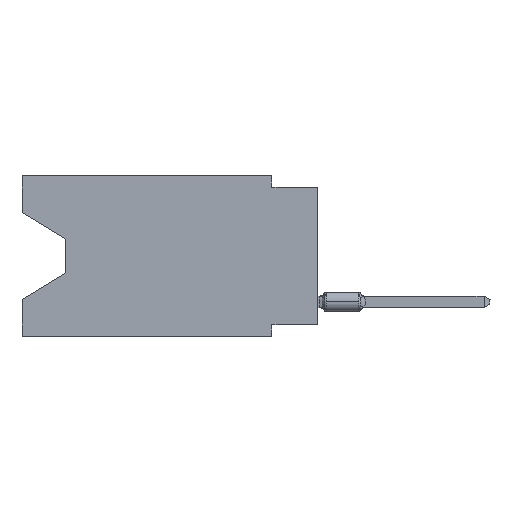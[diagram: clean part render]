
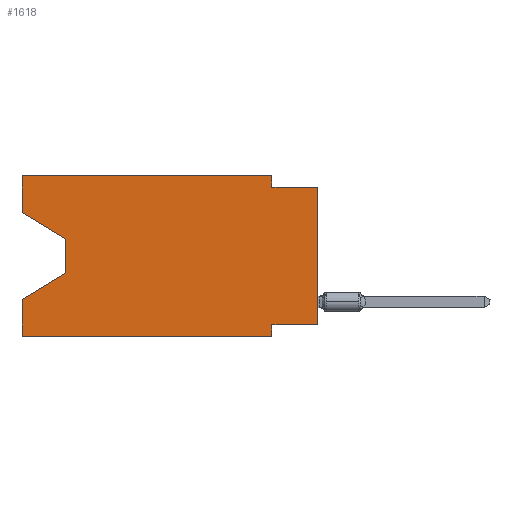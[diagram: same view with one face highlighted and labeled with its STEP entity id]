
A CAD part, left-side view. The second image highlights one B-rep face of the part: STEP entity #1618.
In plain terms, the highlighted planar face has unit normal (-1, 0, 0).
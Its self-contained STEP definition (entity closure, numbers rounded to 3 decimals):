
#298 = VECTOR ( 'NONE', #30956, 1000. ) ;
#580 = CARTESIAN_POINT ( 'NONE',  ( 0., 0., -8.255 ) ) ;
#858 = ORIENTED_EDGE ( 'NONE', *, *, #6671, .F. ) ;
#886 = VECTOR ( 'NONE', #31350, 1000. ) ;
#1618 = ADVANCED_FACE ( 'NONE', ( #19046 ), #13913, .F. ) ;
#1957 = ORIENTED_EDGE ( 'NONE', *, *, #16090, .F. ) ;
#2013 = EDGE_CURVE ( 'NONE', #16493, #16720, #28069, .T. ) ;
#2426 = DIRECTION ( 'NONE',  ( 0., -1., 0. ) ) ;
#2640 = ORIENTED_EDGE ( 'NONE', *, *, #2013, .F. ) ;
#3637 = DIRECTION ( 'NONE',  ( 0., 1., 0. ) ) ;
#3791 = VERTEX_POINT ( 'NONE', #17957 ) ;
#4318 = CARTESIAN_POINT ( 'NONE',  ( 0., 2.54, -8.89 ) ) ;
#4594 = CARTESIAN_POINT ( 'NONE',  ( 0., 16.383, 0. ) ) ;
#5407 = LINE ( 'NONE', #37111, #23847 ) ;
#6587 = LINE ( 'NONE', #32615, #25284 ) ;
#6671 = EDGE_CURVE ( 'NONE', #9391, #3791, #11641, .T. ) ;
#6798 = CARTESIAN_POINT ( 'NONE',  ( 0., 16.383, -2.038 ) ) ;
#7150 = VECTOR ( 'NONE', #18916, 1000. ) ;
#7283 = EDGE_CURVE ( 'NONE', #34559, #29490, #18613, .T. ) ;
#7591 = CARTESIAN_POINT ( 'NONE',  ( 0., 16.383, 0. ) ) ;
#7756 = CARTESIAN_POINT ( 'NONE',  ( 0., 16.383, 0. ) ) ;
#8156 = LINE ( 'NONE', #19730, #886 ) ;
#8918 = EDGE_CURVE ( 'NONE', #21705, #3791, #13652, .T. ) ;
#8978 = CARTESIAN_POINT ( 'NONE',  ( 0., 2.54, -0.635 ) ) ;
#9054 = DIRECTION ( 'NONE',  ( 0., -0.855, -0.519 ) ) ;
#9391 = VERTEX_POINT ( 'NONE', #34723 ) ;
#9817 = EDGE_CURVE ( 'NONE', #34559, #28763, #8156, .T. ) ;
#9829 = LINE ( 'NONE', #19803, #34940 ) ;
#10849 = ORIENTED_EDGE ( 'NONE', *, *, #15200, .F. ) ;
#10994 = DIRECTION ( 'NONE',  ( 0., 0.855, -0.519 ) ) ;
#11641 = LINE ( 'NONE', #17142, #26912 ) ;
#12891 = VECTOR ( 'NONE', #16173, 1000. ) ;
#13652 = LINE ( 'NONE', #25256, #19623 ) ;
#13913 = PLANE ( 'NONE',  #17559 ) ;
#13921 = VERTEX_POINT ( 'NONE', #23879 ) ;
#14671 = CARTESIAN_POINT ( 'NONE',  ( 0., 13.97, -3.505 ) ) ;
#15200 = EDGE_CURVE ( 'NONE', #19103, #16493, #25244, .T. ) ;
#15353 = VECTOR ( 'NONE', #21199, 1000. ) ;
#16023 = EDGE_CURVE ( 'NONE', #16579, #28763, #30318, .T. ) ;
#16090 = EDGE_CURVE ( 'NONE', #16720, #16579, #5407, .T. ) ;
#16173 = DIRECTION ( 'NONE',  ( 0., 0., -1. ) ) ;
#16197 = DIRECTION ( 'NONE',  ( 0., 0., -1. ) ) ;
#16493 = VERTEX_POINT ( 'NONE', #4594 ) ;
#16579 = VERTEX_POINT ( 'NONE', #8978 ) ;
#16720 = VERTEX_POINT ( 'NONE', #35563 ) ;
#17142 = CARTESIAN_POINT ( 'NONE',  ( 0., 16.383, 0. ) ) ;
#17451 = ORIENTED_EDGE ( 'NONE', *, *, #8918, .T. ) ;
#17559 = AXIS2_PLACEMENT_3D ( 'NONE', #30648, #27982, #16197 ) ;
#17957 = CARTESIAN_POINT ( 'NONE',  ( 0., 16.383, -6.852 ) ) ;
#18613 = LINE ( 'NONE', #580, #35452 ) ;
#18916 = DIRECTION ( 'NONE',  ( 0., 0., -1. ) ) ;
#19046 = FACE_OUTER_BOUND ( 'NONE', #34073, .T. ) ;
#19103 = VERTEX_POINT ( 'NONE', #6798 ) ;
#19299 = EDGE_CURVE ( 'NONE', #9391, #13921, #9829, .T. ) ;
#19623 = VECTOR ( 'NONE', #10994, 1000. ) ;
#19730 = CARTESIAN_POINT ( 'NONE',  ( 0., 0., 0. ) ) ;
#19803 = CARTESIAN_POINT ( 'NONE',  ( 0., 16.383, -8.89 ) ) ;
#20292 = ORIENTED_EDGE ( 'NONE', *, *, #21709, .T. ) ;
#20627 = CARTESIAN_POINT ( 'NONE',  ( 0., 0., -8.255 ) ) ;
#20855 = EDGE_CURVE ( 'NONE', #19103, #23430, #6587, .T. ) ;
#20879 = ORIENTED_EDGE ( 'NONE', *, *, #16023, .F. ) ;
#21199 = DIRECTION ( 'NONE',  ( 0., -1., 0. ) ) ;
#21396 = ORIENTED_EDGE ( 'NONE', *, *, #7283, .F. ) ;
#21564 = VECTOR ( 'NONE', #2426, 1000. ) ;
#21705 = VERTEX_POINT ( 'NONE', #24381 ) ;
#21709 = EDGE_CURVE ( 'NONE', #23430, #21705, #33665, .T. ) ;
#23430 = VERTEX_POINT ( 'NONE', #14671 ) ;
#23431 = DIRECTION ( 'NONE',  ( 0., 0., 1. ) ) ;
#23847 = VECTOR ( 'NONE', #28581, 1000. ) ;
#23879 = CARTESIAN_POINT ( 'NONE',  ( 0., 2.54, -8.89 ) ) ;
#24381 = CARTESIAN_POINT ( 'NONE',  ( 0., 13.97, -5.385 ) ) ;
#24425 = CARTESIAN_POINT ( 'NONE',  ( 0., 0., -0.635 ) ) ;
#24445 = DIRECTION ( 'NONE',  ( 0., -1., 0. ) ) ;
#24885 = ORIENTED_EDGE ( 'NONE', *, *, #34233, .F. ) ;
#25244 = LINE ( 'NONE', #7591, #298 ) ;
#25256 = CARTESIAN_POINT ( 'NONE',  ( 0., 13.97, -5.385 ) ) ;
#25284 = VECTOR ( 'NONE', #9054, 1000. ) ;
#26912 = VECTOR ( 'NONE', #23431, 1000. ) ;
#27629 = CARTESIAN_POINT ( 'NONE',  ( 0., 2.54, -8.255 ) ) ;
#27982 = DIRECTION ( 'NONE',  ( 1., 0., 0. ) ) ;
#28069 = LINE ( 'NONE', #7756, #21564 ) ;
#28581 = DIRECTION ( 'NONE',  ( 0., 0., -1. ) ) ;
#28763 = VERTEX_POINT ( 'NONE', #36815 ) ;
#29490 = VERTEX_POINT ( 'NONE', #27629 ) ;
#29682 = ORIENTED_EDGE ( 'NONE', *, *, #19299, .T. ) ;
#30318 = LINE ( 'NONE', #24425, #15353 ) ;
#30348 = LINE ( 'NONE', #4318, #7150 ) ;
#30648 = CARTESIAN_POINT ( 'NONE',  ( 0., 16.383, 0. ) ) ;
#30956 = DIRECTION ( 'NONE',  ( 0., 0., 1. ) ) ;
#31350 = DIRECTION ( 'NONE',  ( 0., 0., 1. ) ) ;
#32615 = CARTESIAN_POINT ( 'NONE',  ( 0., 16.383, -2.038 ) ) ;
#33665 = LINE ( 'NONE', #35960, #12891 ) ;
#34073 = EDGE_LOOP ( 'NONE', ( #34451, #20292, #17451, #858, #29682, #24885, #21396, #35978, #20879, #1957, #2640, #10849 ) ) ;
#34233 = EDGE_CURVE ( 'NONE', #29490, #13921, #30348, .T. ) ;
#34451 = ORIENTED_EDGE ( 'NONE', *, *, #20855, .T. ) ;
#34559 = VERTEX_POINT ( 'NONE', #20627 ) ;
#34723 = CARTESIAN_POINT ( 'NONE',  ( 0., 16.383, -8.89 ) ) ;
#34940 = VECTOR ( 'NONE', #24445, 1000. ) ;
#35452 = VECTOR ( 'NONE', #3637, 1000. ) ;
#35563 = CARTESIAN_POINT ( 'NONE',  ( 0., 2.54, 0. ) ) ;
#35960 = CARTESIAN_POINT ( 'NONE',  ( 0., 13.97, -3.505 ) ) ;
#35978 = ORIENTED_EDGE ( 'NONE', *, *, #9817, .T. ) ;
#36815 = CARTESIAN_POINT ( 'NONE',  ( 0., 0., -0.635 ) ) ;
#37111 = CARTESIAN_POINT ( 'NONE',  ( 0., 2.54, 0. ) ) ;
